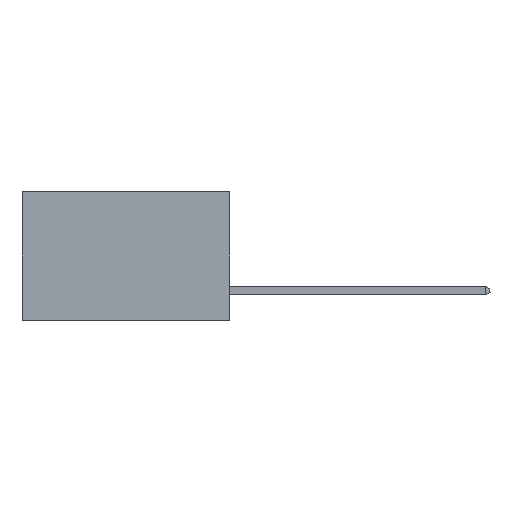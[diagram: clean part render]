
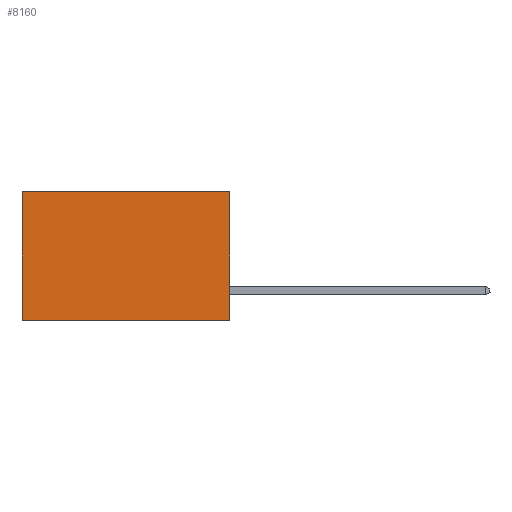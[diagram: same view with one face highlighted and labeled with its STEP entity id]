
A CAD part, left-side view. The second image highlights one B-rep face of the part: STEP entity #8160.
In plain terms, the highlighted planar face has unit normal (-1, 0, 0).
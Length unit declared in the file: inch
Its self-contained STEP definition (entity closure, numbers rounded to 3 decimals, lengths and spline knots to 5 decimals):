
#66 = LINE ( 'NONE', #29871, #14768 ) ;
#460 = CARTESIAN_POINT ( 'NONE',  ( 0.298, 0., -0.37 ) ) ;
#3278 = CARTESIAN_POINT ( 'NONE',  ( 0.298, 0., 0. ) ) ;
#4285 = ORIENTED_EDGE ( 'NONE', *, *, #19171, .T. ) ;
#5371 = VERTEX_POINT ( 'NONE', #26170 ) ;
#5394 = ORIENTED_EDGE ( 'NONE', *, *, #27480, .F. ) ;
#5784 = PLANE ( 'NONE',  #18472 ) ;
#6002 = CARTESIAN_POINT ( 'NONE',  ( 0.298, 0.6, 0. ) ) ;
#8060 = CARTESIAN_POINT ( 'NONE',  ( 0.298, 0.6, -0.37 ) ) ;
#8160 = ADVANCED_FACE ( 'NONE', ( #17099 ), #5784, .F. ) ;
#8380 = LINE ( 'NONE', #14126, #9839 ) ;
#8669 = DIRECTION ( 'NONE',  ( 0., 1., 0. ) ) ;
#9746 = LINE ( 'NONE', #21187, #24015 ) ;
#9839 = VECTOR ( 'NONE', #24011, 39.37008 ) ;
#10355 = VERTEX_POINT ( 'NONE', #8060 ) ;
#10367 = CARTESIAN_POINT ( 'NONE',  ( 0.298, 0., 0. ) ) ;
#14126 = CARTESIAN_POINT ( 'NONE',  ( 0.298, 0., -0.37 ) ) ;
#14473 = VECTOR ( 'NONE', #8669, 39.37008 ) ;
#14768 = VECTOR ( 'NONE', #15903, 39.37008 ) ;
#15903 = DIRECTION ( 'NONE',  ( 0., 0., -1. ) ) ;
#16367 = ORIENTED_EDGE ( 'NONE', *, *, #17251, .F. ) ;
#17099 = FACE_OUTER_BOUND ( 'NONE', #22602, .T. ) ;
#17251 = EDGE_CURVE ( 'NONE', #5371, #27546, #9746, .T. ) ;
#17891 = EDGE_CURVE ( 'NONE', #5371, #18856, #20683, .T. ) ;
#18472 = AXIS2_PLACEMENT_3D ( 'NONE', #10367, #19804, #21868 ) ;
#18856 = VERTEX_POINT ( 'NONE', #6002 ) ;
#19123 = ORIENTED_EDGE ( 'NONE', *, *, #17891, .T. ) ;
#19171 = EDGE_CURVE ( 'NONE', #18856, #10355, #66, .T. ) ;
#19804 = DIRECTION ( 'NONE',  ( 1., 0., 0. ) ) ;
#20683 = LINE ( 'NONE', #3278, #14473 ) ;
#21187 = CARTESIAN_POINT ( 'NONE',  ( 0.298, 0., 0. ) ) ;
#21868 = DIRECTION ( 'NONE',  ( 0., 0., -1. ) ) ;
#22602 = EDGE_LOOP ( 'NONE', ( #4285, #5394, #16367, #19123 ) ) ;
#24011 = DIRECTION ( 'NONE',  ( 0., 1., 0. ) ) ;
#24015 = VECTOR ( 'NONE', #25961, 39.37008 ) ;
#25961 = DIRECTION ( 'NONE',  ( 0., 0., -1. ) ) ;
#26170 = CARTESIAN_POINT ( 'NONE',  ( 0.298, 0., 0. ) ) ;
#27480 = EDGE_CURVE ( 'NONE', #27546, #10355, #8380, .T. ) ;
#27546 = VERTEX_POINT ( 'NONE', #460 ) ;
#29871 = CARTESIAN_POINT ( 'NONE',  ( 0.298, 0.6, 0. ) ) ;
